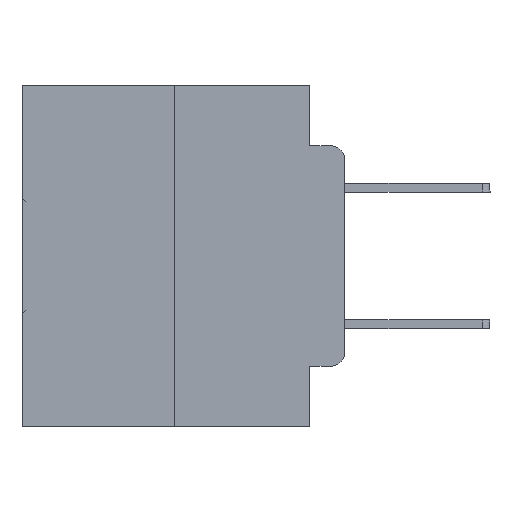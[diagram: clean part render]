
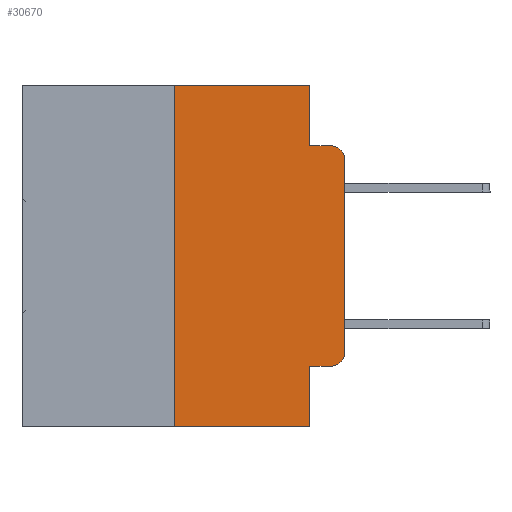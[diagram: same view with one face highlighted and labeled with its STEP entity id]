
A CAD part, left-side view. The second image highlights one B-rep face of the part: STEP entity #30670.
In plain terms, the highlighted planar face has unit normal (-1, 0, 0).
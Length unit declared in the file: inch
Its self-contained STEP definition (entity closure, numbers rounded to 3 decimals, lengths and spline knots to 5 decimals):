
#690 = VECTOR ( 'NONE', #15099, 39.37008 ) ;
#842 = ORIENTED_EDGE ( 'NONE', *, *, #9501, .F. ) ;
#1013 = VECTOR ( 'NONE', #10747, 39.37008 ) ;
#1226 = ORIENTED_EDGE ( 'NONE', *, *, #28062, .T. ) ;
#1471 = LINE ( 'NONE', #24191, #27620 ) ;
#1561 = AXIS2_PLACEMENT_3D ( 'NONE', #13251, #30783, #15791 ) ;
#2476 = ORIENTED_EDGE ( 'NONE', *, *, #6092, .T. ) ;
#2526 = LINE ( 'NONE', #22342, #9325 ) ;
#2669 = VERTEX_POINT ( 'NONE', #29307 ) ;
#2994 = CARTESIAN_POINT ( 'NONE',  ( 0., 0.051, 0. ) ) ;
#3465 = CARTESIAN_POINT ( 'NONE',  ( 0., 0.473, -0.5 ) ) ;
#3613 = CARTESIAN_POINT ( 'NONE',  ( 0., 0.473, 0. ) ) ;
#3792 = CARTESIAN_POINT ( 'NONE',  ( 0., 0., -0.3915 ) ) ;
#3961 = DIRECTION ( 'NONE',  ( 0., -1., 0. ) ) ;
#4159 = EDGE_CURVE ( 'NONE', #9498, #9709, #27463, .T. ) ;
#4498 = CARTESIAN_POINT ( 'NONE',  ( 0., 0.02, -0.3915 ) ) ;
#5409 = CARTESIAN_POINT ( 'NONE',  ( 0., 0.02, -0.0885 ) ) ;
#6092 = EDGE_CURVE ( 'NONE', #31873, #7094, #22196, .T. ) ;
#6993 = CARTESIAN_POINT ( 'NONE',  ( 0., 0.051, -0.5 ) ) ;
#7083 = DIRECTION ( 'NONE',  ( 0., 0., -1. ) ) ;
#7094 = VERTEX_POINT ( 'NONE', #3792 ) ;
#7247 = DIRECTION ( 'NONE',  ( 0., -1., 0. ) ) ;
#7810 = EDGE_CURVE ( 'NONE', #29007, #31873, #1471, .T. ) ;
#9325 = VECTOR ( 'NONE', #7247, 39.37008 ) ;
#9395 = DIRECTION ( 'NONE',  ( 0., 0., -1. ) ) ;
#9498 = VERTEX_POINT ( 'NONE', #31195 ) ;
#9501 = EDGE_CURVE ( 'NONE', #29007, #9709, #30608, .T. ) ;
#9709 = VERTEX_POINT ( 'NONE', #6993 ) ;
#10222 = EDGE_CURVE ( 'NONE', #12511, #30600, #24303, .T. ) ;
#10506 = ORIENTED_EDGE ( 'NONE', *, *, #17967, .F. ) ;
#10747 = DIRECTION ( 'NONE',  ( 0., 0., -1. ) ) ;
#11202 = DIRECTION ( 'NONE',  ( 0., -1., 0. ) ) ;
#11283 = DIRECTION ( 'NONE',  ( 0., 0., -1. ) ) ;
#11776 = FACE_OUTER_BOUND ( 'NONE', #28426, .T. ) ;
#12511 = VERTEX_POINT ( 'NONE', #29569 ) ;
#13251 = CARTESIAN_POINT ( 'NONE',  ( 0., 0.02, -0.1085 ) ) ;
#13456 = DIRECTION ( 'NONE',  ( 0., 0., 1. ) ) ;
#14100 = VECTOR ( 'NONE', #11202, 39.37008 ) ;
#14438 = ORIENTED_EDGE ( 'NONE', *, *, #7810, .T. ) ;
#14819 = ORIENTED_EDGE ( 'NONE', *, *, #19626, .F. ) ;
#15099 = DIRECTION ( 'NONE',  ( 0., 0., 1. ) ) ;
#15791 = DIRECTION ( 'NONE',  ( 0., 0., -1. ) ) ;
#16292 = EDGE_CURVE ( 'NONE', #9498, #12511, #21727, .T. ) ;
#17967 = EDGE_CURVE ( 'NONE', #30600, #2669, #21254, .T. ) ;
#18179 = VERTEX_POINT ( 'NONE', #19025 ) ;
#19025 = CARTESIAN_POINT ( 'NONE',  ( 0., 0., -0.1085 ) ) ;
#19191 = CARTESIAN_POINT ( 'NONE',  ( 0., 0.051, 0. ) ) ;
#19438 = AXIS2_PLACEMENT_3D ( 'NONE', #4498, #22179, #7083 ) ;
#19510 = ORIENTED_EDGE ( 'NONE', *, *, #16292, .F. ) ;
#19626 = EDGE_CURVE ( 'NONE', #2669, #22091, #2526, .T. ) ;
#20307 = ORIENTED_EDGE ( 'NONE', *, *, #4159, .T. ) ;
#21254 = LINE ( 'NONE', #2994, #1013 ) ;
#21296 = DIRECTION ( 'NONE',  ( 0., -1., 0. ) ) ;
#21727 = LINE ( 'NONE', #25186, #690 ) ;
#22091 = VERTEX_POINT ( 'NONE', #5409 ) ;
#22179 = DIRECTION ( 'NONE',  ( -1., 0., 0. ) ) ;
#22196 = CIRCLE ( 'NONE', #19438, 0.02 ) ;
#22342 = CARTESIAN_POINT ( 'NONE',  ( 0., 0.051, -0.0885 ) ) ;
#22410 = CARTESIAN_POINT ( 'NONE',  ( 0., 0.02, -0.4115 ) ) ;
#23959 = VECTOR ( 'NONE', #11283, 39.37008 ) ;
#24191 = CARTESIAN_POINT ( 'NONE',  ( 0., 0.051, -0.4115 ) ) ;
#24303 = LINE ( 'NONE', #3613, #30948 ) ;
#24481 = DIRECTION ( 'NONE',  ( 1., 0., 0. ) ) ;
#25186 = CARTESIAN_POINT ( 'NONE',  ( 0., 0.25, 0. ) ) ;
#25196 = LINE ( 'NONE', #25982, #31043 ) ;
#25432 = ORIENTED_EDGE ( 'NONE', *, *, #10222, .F. ) ;
#25982 = CARTESIAN_POINT ( 'NONE',  ( 0., 0., 0. ) ) ;
#26591 = ORIENTED_EDGE ( 'NONE', *, *, #29722, .T. ) ;
#26893 = CARTESIAN_POINT ( 'NONE',  ( 0., 0.473, 0. ) ) ;
#27066 = AXIS2_PLACEMENT_3D ( 'NONE', #26893, #24481, #9395 ) ;
#27463 = LINE ( 'NONE', #3465, #14100 ) ;
#27620 = VECTOR ( 'NONE', #3961, 39.37008 ) ;
#28062 = EDGE_CURVE ( 'NONE', #18179, #22091, #28322, .T. ) ;
#28322 = CIRCLE ( 'NONE', #1561, 0.02 ) ;
#28426 = EDGE_LOOP ( 'NONE', ( #26591, #1226, #14819, #10506, #25432, #19510, #20307, #842, #14438, #2476 ) ) ;
#29007 = VERTEX_POINT ( 'NONE', #30179 ) ;
#29307 = CARTESIAN_POINT ( 'NONE',  ( 0., 0.051, -0.0885 ) ) ;
#29569 = CARTESIAN_POINT ( 'NONE',  ( 0., 0.25, 0. ) ) ;
#29722 = EDGE_CURVE ( 'NONE', #7094, #18179, #25196, .T. ) ;
#30179 = CARTESIAN_POINT ( 'NONE',  ( 0., 0.051, -0.4115 ) ) ;
#30600 = VERTEX_POINT ( 'NONE', #19191 ) ;
#30608 = LINE ( 'NONE', #31306, #23959 ) ;
#30670 = ADVANCED_FACE ( 'NONE', ( #11776 ), #31876, .F. ) ;
#30783 = DIRECTION ( 'NONE',  ( -1., 0., 0. ) ) ;
#30948 = VECTOR ( 'NONE', #21296, 39.37008 ) ;
#31043 = VECTOR ( 'NONE', #13456, 39.37008 ) ;
#31195 = CARTESIAN_POINT ( 'NONE',  ( 0., 0.25, -0.5 ) ) ;
#31306 = CARTESIAN_POINT ( 'NONE',  ( 0., 0.051, 0. ) ) ;
#31873 = VERTEX_POINT ( 'NONE', #22410 ) ;
#31876 = PLANE ( 'NONE',  #27066 ) ;
